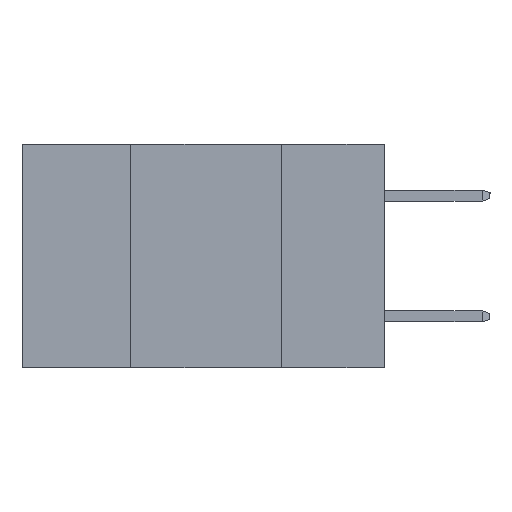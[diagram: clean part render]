
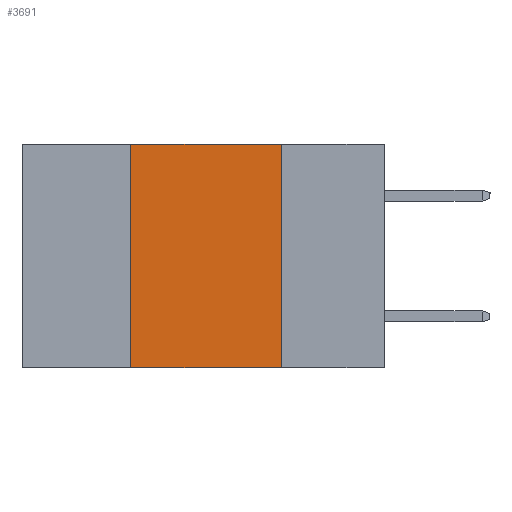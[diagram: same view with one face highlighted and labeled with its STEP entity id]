
A CAD part, left-side view. The second image highlights one B-rep face of the part: STEP entity #3691.
In plain terms, the highlighted planar face has unit normal (-1, 0, 0).
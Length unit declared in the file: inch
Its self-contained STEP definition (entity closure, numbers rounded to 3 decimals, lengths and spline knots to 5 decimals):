
#21 = CARTESIAN_POINT ( 'NONE',  ( 0., 0.17, -0.37 ) ) ;
#241 = LINE ( 'NONE', #6497, #6584 ) ;
#983 = EDGE_LOOP ( 'NONE', ( #5941, #8505, #8256, #3487 ) ) ;
#1214 = CARTESIAN_POINT ( 'NONE',  ( 0., 0.6, -0.37 ) ) ;
#1241 = PLANE ( 'NONE',  #6051 ) ;
#1767 = VECTOR ( 'NONE', #1899, 39.37008 ) ;
#1899 = DIRECTION ( 'NONE',  ( 0., 0., -1. ) ) ;
#1977 = CARTESIAN_POINT ( 'NONE',  ( 0., 0.6, 0. ) ) ;
#3033 = CARTESIAN_POINT ( 'NONE',  ( 0., 0.17, 0. ) ) ;
#3291 = EDGE_CURVE ( 'NONE', #4685, #5101, #4901, .T. ) ;
#3487 = ORIENTED_EDGE ( 'NONE', *, *, #9524, .T. ) ;
#3691 = ADVANCED_FACE ( 'NONE', ( #8602 ), #1241, .F. ) ;
#3865 = LINE ( 'NONE', #6636, #4389 ) ;
#4084 = EDGE_CURVE ( 'NONE', #4456, #4685, #241, .T. ) ;
#4244 = DIRECTION ( 'NONE',  ( 0., -1., 0. ) ) ;
#4325 = CARTESIAN_POINT ( 'NONE',  ( 0., 0.42, 0. ) ) ;
#4389 = VECTOR ( 'NONE', #6918, 39.37008 ) ;
#4456 = VERTEX_POINT ( 'NONE', #4325 ) ;
#4685 = VERTEX_POINT ( 'NONE', #3033 ) ;
#4901 = LINE ( 'NONE', #7922, #1767 ) ;
#5034 = DIRECTION ( 'NONE',  ( 0., 0., -1. ) ) ;
#5101 = VERTEX_POINT ( 'NONE', #21 ) ;
#5324 = CARTESIAN_POINT ( 'NONE',  ( 0., 0.42, -0.37 ) ) ;
#5639 = DIRECTION ( 'NONE',  ( 1., 0., 0. ) ) ;
#5941 = ORIENTED_EDGE ( 'NONE', *, *, #3291, .F. ) ;
#6048 = VERTEX_POINT ( 'NONE', #5324 ) ;
#6051 = AXIS2_PLACEMENT_3D ( 'NONE', #1977, #5639, #5034 ) ;
#6487 = VECTOR ( 'NONE', #4244, 39.37008 ) ;
#6497 = CARTESIAN_POINT ( 'NONE',  ( 0., 0.6, 0. ) ) ;
#6584 = VECTOR ( 'NONE', #7272, 39.37008 ) ;
#6636 = CARTESIAN_POINT ( 'NONE',  ( 0., 0.42, -0.37 ) ) ;
#6918 = DIRECTION ( 'NONE',  ( 0., 0., 1. ) ) ;
#7272 = DIRECTION ( 'NONE',  ( 0., -1., 0. ) ) ;
#7373 = LINE ( 'NONE', #1214, #6487 ) ;
#7922 = CARTESIAN_POINT ( 'NONE',  ( 0., 0.17, -0.37 ) ) ;
#8256 = ORIENTED_EDGE ( 'NONE', *, *, #8399, .F. ) ;
#8399 = EDGE_CURVE ( 'NONE', #6048, #4456, #3865, .T. ) ;
#8505 = ORIENTED_EDGE ( 'NONE', *, *, #4084, .F. ) ;
#8602 = FACE_OUTER_BOUND ( 'NONE', #983, .T. ) ;
#9524 = EDGE_CURVE ( 'NONE', #6048, #5101, #7373, .T. ) ;
